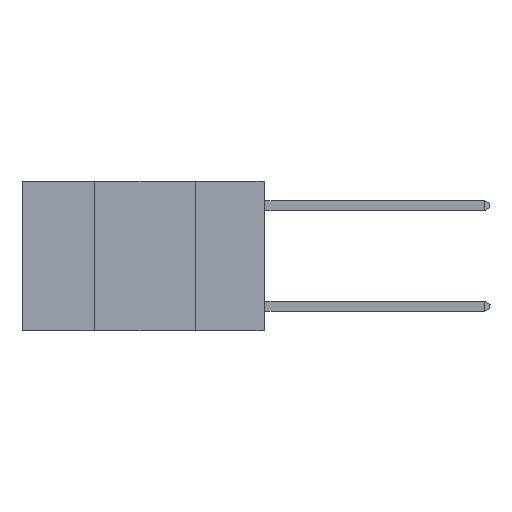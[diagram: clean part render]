
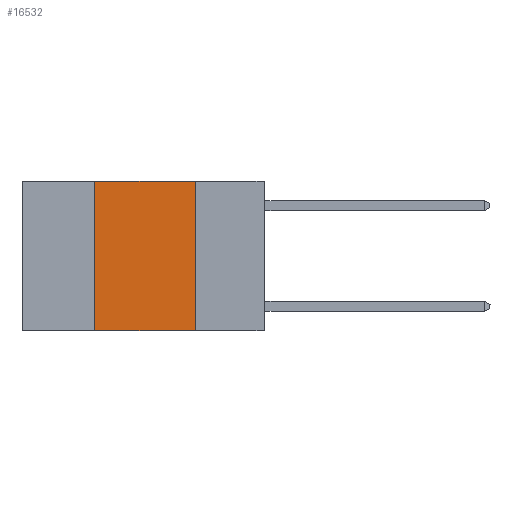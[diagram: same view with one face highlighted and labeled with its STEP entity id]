
A CAD part, left-side view. The second image highlights one B-rep face of the part: STEP entity #16532.
In plain terms, the highlighted planar face has unit normal (-1, 0, 0).
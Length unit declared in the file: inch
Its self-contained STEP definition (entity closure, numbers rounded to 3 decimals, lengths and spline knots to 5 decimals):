
#232 = DIRECTION ( 'NONE',  ( 0., -1., 0. ) ) ;
#555 = FACE_OUTER_BOUND ( 'NONE', #1344, .T. ) ;
#1274 = CARTESIAN_POINT ( 'NONE',  ( 0., 0.17, 0. ) ) ;
#1344 = EDGE_LOOP ( 'NONE', ( #3922, #4431, #3186, #17730 ) ) ;
#1872 = VECTOR ( 'NONE', #5245, 39.37008 ) ;
#2378 = LINE ( 'NONE', #8430, #1872 ) ;
#2734 = PLANE ( 'NONE',  #10275 ) ;
#3186 = ORIENTED_EDGE ( 'NONE', *, *, #8688, .F. ) ;
#3922 = ORIENTED_EDGE ( 'NONE', *, *, #9128, .F. ) ;
#3932 = VECTOR ( 'NONE', #19064, 39.37008 ) ;
#4431 = ORIENTED_EDGE ( 'NONE', *, *, #16164, .F. ) ;
#5099 = CARTESIAN_POINT ( 'NONE',  ( 0., 0.6, 0. ) ) ;
#5245 = DIRECTION ( 'NONE',  ( 0., 0., -1. ) ) ;
#6304 = VERTEX_POINT ( 'NONE', #1274 ) ;
#6553 = VERTEX_POINT ( 'NONE', #18894 ) ;
#6608 = CARTESIAN_POINT ( 'NONE',  ( 0., 0.42, 0. ) ) ;
#7625 = DIRECTION ( 'NONE',  ( 1., 0., 0. ) ) ;
#7707 = VECTOR ( 'NONE', #232, 39.37008 ) ;
#8430 = CARTESIAN_POINT ( 'NONE',  ( 0., 0.17, 0. ) ) ;
#8608 = EDGE_CURVE ( 'NONE', #16697, #6553, #14514, .T. ) ;
#8688 = EDGE_CURVE ( 'NONE', #16697, #16123, #12197, .T. ) ;
#9128 = EDGE_CURVE ( 'NONE', #6304, #6553, #2378, .T. ) ;
#9613 = CARTESIAN_POINT ( 'NONE',  ( 0., 0.42, -0.37 ) ) ;
#10275 = AXIS2_PLACEMENT_3D ( 'NONE', #16566, #7625, #17990 ) ;
#11539 = CARTESIAN_POINT ( 'NONE',  ( 0., 0.6, -0.37 ) ) ;
#11710 = LINE ( 'NONE', #5099, #7707 ) ;
#12197 = LINE ( 'NONE', #17601, #3932 ) ;
#14050 = VECTOR ( 'NONE', #16003, 39.37008 ) ;
#14514 = LINE ( 'NONE', #11539, #14050 ) ;
#16003 = DIRECTION ( 'NONE',  ( 0., -1., 0. ) ) ;
#16123 = VERTEX_POINT ( 'NONE', #6608 ) ;
#16164 = EDGE_CURVE ( 'NONE', #16123, #6304, #11710, .T. ) ;
#16532 = ADVANCED_FACE ( 'NONE', ( #555 ), #2734, .F. ) ;
#16566 = CARTESIAN_POINT ( 'NONE',  ( 0., 0.6, 0. ) ) ;
#16697 = VERTEX_POINT ( 'NONE', #9613 ) ;
#17601 = CARTESIAN_POINT ( 'NONE',  ( 0., 0.42, 0. ) ) ;
#17730 = ORIENTED_EDGE ( 'NONE', *, *, #8608, .T. ) ;
#17990 = DIRECTION ( 'NONE',  ( 0., 0., -1. ) ) ;
#18894 = CARTESIAN_POINT ( 'NONE',  ( 0., 0.17, -0.37 ) ) ;
#19064 = DIRECTION ( 'NONE',  ( 0., 0., 1. ) ) ;
